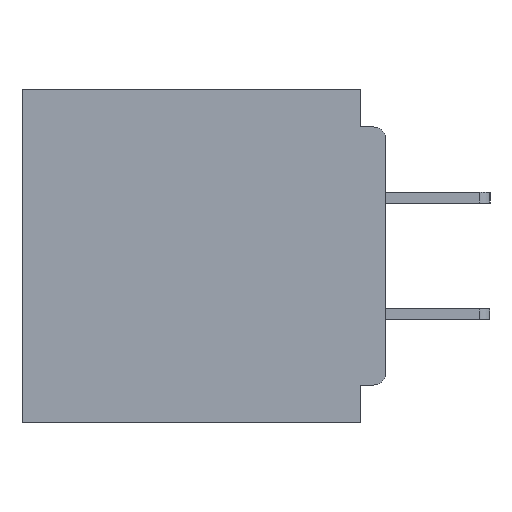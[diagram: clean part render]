
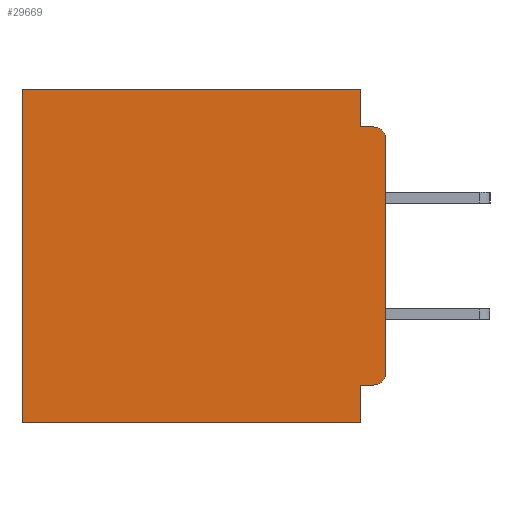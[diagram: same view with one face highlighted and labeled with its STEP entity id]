
A CAD part, left-side view. The second image highlights one B-rep face of the part: STEP entity #29669.
In plain terms, the highlighted planar face has unit normal (-1, 0, 0).
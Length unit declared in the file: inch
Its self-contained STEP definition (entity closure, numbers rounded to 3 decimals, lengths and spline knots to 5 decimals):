
#541 = VECTOR ( 'NONE', #30825, 39.37008 ) ;
#734 = VERTEX_POINT ( 'NONE', #14045 ) ;
#858 = ORIENTED_EDGE ( 'NONE', *, *, #38944, .F. ) ;
#1121 = DIRECTION ( 'NONE',  ( 0., 0., -1. ) ) ;
#4493 = VERTEX_POINT ( 'NONE', #36590 ) ;
#4813 = AXIS2_PLACEMENT_3D ( 'NONE', #18136, #21543, #1121 ) ;
#5238 = ORIENTED_EDGE ( 'NONE', *, *, #31674, .F. ) ;
#5488 = LINE ( 'NONE', #35113, #13484 ) ;
#5746 = ORIENTED_EDGE ( 'NONE', *, *, #24990, .F. ) ;
#6683 = CARTESIAN_POINT ( 'NONE',  ( 0.3, 0.031, 0. ) ) ;
#8377 = CARTESIAN_POINT ( 'NONE',  ( 0.3, 0., -0.34 ) ) ;
#8453 = ORIENTED_EDGE ( 'NONE', *, *, #34311, .F. ) ;
#8566 = CARTESIAN_POINT ( 'NONE',  ( 0.3, 0.437, 0. ) ) ;
#8697 = CARTESIAN_POINT ( 'NONE',  ( 0.3, 0.031, -0.045 ) ) ;
#8823 = CARTESIAN_POINT ( 'NONE',  ( 0.3, 0.437, -0.4 ) ) ;
#8952 = VECTOR ( 'NONE', #42684, 39.37008 ) ;
#9533 = ORIENTED_EDGE ( 'NONE', *, *, #34887, .T. ) ;
#10636 = EDGE_CURVE ( 'NONE', #12617, #14542, #21453, .T. ) ;
#11389 = PLANE ( 'NONE',  #4813 ) ;
#11642 = ORIENTED_EDGE ( 'NONE', *, *, #10636, .T. ) ;
#12617 = VERTEX_POINT ( 'NONE', #23183 ) ;
#13241 = ORIENTED_EDGE ( 'NONE', *, *, #29785, .T. ) ;
#13242 = AXIS2_PLACEMENT_3D ( 'NONE', #34370, #14062, #37816 ) ;
#13332 = DIRECTION ( 'NONE',  ( 0., 0., -1. ) ) ;
#13484 = VECTOR ( 'NONE', #25001, 39.37008 ) ;
#13525 = CARTESIAN_POINT ( 'NONE',  ( 0.3, 0.015, -0.355 ) ) ;
#13835 = CARTESIAN_POINT ( 'NONE',  ( 0.3, 0.015, -0.06 ) ) ;
#14045 = CARTESIAN_POINT ( 'NONE',  ( 0.3, 0.437, -0.4 ) ) ;
#14062 = DIRECTION ( 'NONE',  ( -1., 0., 0. ) ) ;
#14542 = VERTEX_POINT ( 'NONE', #29185 ) ;
#14864 = AXIS2_PLACEMENT_3D ( 'NONE', #13835, #37586, #17231 ) ;
#14909 = FACE_OUTER_BOUND ( 'NONE', #42141, .T. ) ;
#15852 = LINE ( 'NONE', #16905, #41867 ) ;
#16905 = CARTESIAN_POINT ( 'NONE',  ( 0.3, 0., -0.4 ) ) ;
#17231 = DIRECTION ( 'NONE',  ( 0., 0., -1. ) ) ;
#18136 = CARTESIAN_POINT ( 'NONE',  ( 0.3, 0., -0.4 ) ) ;
#18428 = EDGE_CURVE ( 'NONE', #4493, #37706, #34954, .T. ) ;
#18479 = VECTOR ( 'NONE', #37209, 39.37008 ) ;
#18570 = VECTOR ( 'NONE', #19003, 39.37008 ) ;
#18892 = CARTESIAN_POINT ( 'NONE',  ( 0.3, 0.031, -0.4 ) ) ;
#19003 = DIRECTION ( 'NONE',  ( 0., 0., -1. ) ) ;
#19004 = ORIENTED_EDGE ( 'NONE', *, *, #29084, .T. ) ;
#19296 = CARTESIAN_POINT ( 'NONE',  ( 0.3, 0.031, -0.4 ) ) ;
#20565 = VECTOR ( 'NONE', #13332, 39.37008 ) ;
#21453 = CIRCLE ( 'NONE', #14864, 0.015 ) ;
#21543 = DIRECTION ( 'NONE',  ( 1., 0., 0. ) ) ;
#21744 = CARTESIAN_POINT ( 'NONE',  ( 0.3, 0., 0. ) ) ;
#22512 = CIRCLE ( 'NONE', #13242, 0.015 ) ;
#23183 = CARTESIAN_POINT ( 'NONE',  ( 0.3, 0., -0.06 ) ) ;
#24990 = EDGE_CURVE ( 'NONE', #35141, #14542, #27698, .T. ) ;
#25001 = DIRECTION ( 'NONE',  ( 0., 1., 0. ) ) ;
#27056 = CARTESIAN_POINT ( 'NONE',  ( 0.3, 0., -0.4 ) ) ;
#27412 = CARTESIAN_POINT ( 'NONE',  ( 0.3, 0., -0.045 ) ) ;
#27495 = LINE ( 'NONE', #27056, #18479 ) ;
#27698 = LINE ( 'NONE', #27412, #541 ) ;
#29084 = EDGE_CURVE ( 'NONE', #35916, #34424, #40462, .T. ) ;
#29185 = CARTESIAN_POINT ( 'NONE',  ( 0.3, 0.015, -0.045 ) ) ;
#29640 = LINE ( 'NONE', #33610, #20565 ) ;
#29669 = ADVANCED_FACE ( 'NONE', ( #14909 ), #11389, .F. ) ;
#29785 = EDGE_CURVE ( 'NONE', #34424, #734, #36673, .T. ) ;
#30306 = VECTOR ( 'NONE', #31847, 39.37008 ) ;
#30825 = DIRECTION ( 'NONE',  ( 0., -1., 0. ) ) ;
#31674 = EDGE_CURVE ( 'NONE', #37706, #734, #15852, .T. ) ;
#31847 = DIRECTION ( 'NONE',  ( 0., 1., 0. ) ) ;
#33610 = CARTESIAN_POINT ( 'NONE',  ( 0.3, 0.031, 0. ) ) ;
#34311 = EDGE_CURVE ( 'NONE', #38393, #4493, #5488, .T. ) ;
#34370 = CARTESIAN_POINT ( 'NONE',  ( 0.3, 0.015, -0.34 ) ) ;
#34424 = VERTEX_POINT ( 'NONE', #8566 ) ;
#34449 = ORIENTED_EDGE ( 'NONE', *, *, #18428, .F. ) ;
#34887 = EDGE_CURVE ( 'NONE', #38393, #35570, #22512, .T. ) ;
#34954 = LINE ( 'NONE', #18892, #8952 ) ;
#35113 = CARTESIAN_POINT ( 'NONE',  ( 0.3, 0., -0.355 ) ) ;
#35141 = VERTEX_POINT ( 'NONE', #8697 ) ;
#35570 = VERTEX_POINT ( 'NONE', #8377 ) ;
#35916 = VERTEX_POINT ( 'NONE', #6683 ) ;
#36590 = CARTESIAN_POINT ( 'NONE',  ( 0.3, 0.031, -0.355 ) ) ;
#36673 = LINE ( 'NONE', #8823, #18570 ) ;
#37209 = DIRECTION ( 'NONE',  ( 0., 0., -1. ) ) ;
#37586 = DIRECTION ( 'NONE',  ( -1., 0., 0. ) ) ;
#37629 = ORIENTED_EDGE ( 'NONE', *, *, #39059, .F. ) ;
#37706 = VERTEX_POINT ( 'NONE', #19296 ) ;
#37816 = DIRECTION ( 'NONE',  ( 0., 0., -1. ) ) ;
#38393 = VERTEX_POINT ( 'NONE', #13525 ) ;
#38944 = EDGE_CURVE ( 'NONE', #35916, #35141, #29640, .T. ) ;
#39059 = EDGE_CURVE ( 'NONE', #12617, #35570, #27495, .T. ) ;
#40462 = LINE ( 'NONE', #21744, #30306 ) ;
#41867 = VECTOR ( 'NONE', #44041, 39.37008 ) ;
#42141 = EDGE_LOOP ( 'NONE', ( #37629, #11642, #5746, #858, #19004, #13241, #5238, #34449, #8453, #9533 ) ) ;
#42684 = DIRECTION ( 'NONE',  ( 0., 0., -1. ) ) ;
#44041 = DIRECTION ( 'NONE',  ( 0., 1., 0. ) ) ;
